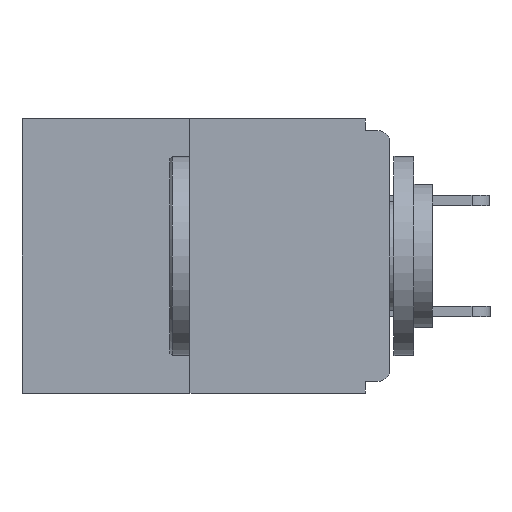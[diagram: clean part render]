
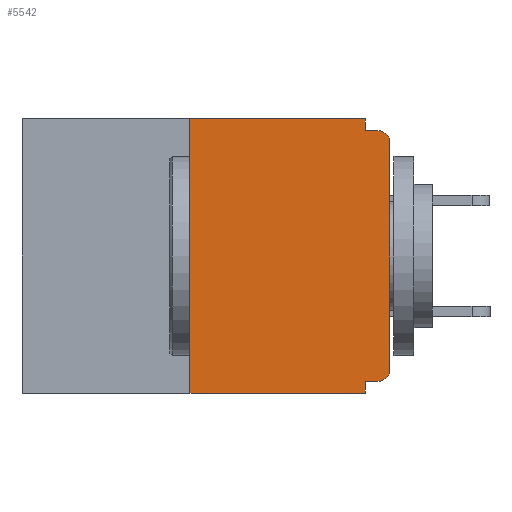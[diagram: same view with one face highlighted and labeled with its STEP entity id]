
A CAD part, left-side view. The second image highlights one B-rep face of the part: STEP entity #5542.
In plain terms, the highlighted planar face has unit normal (-1, 0, 0).
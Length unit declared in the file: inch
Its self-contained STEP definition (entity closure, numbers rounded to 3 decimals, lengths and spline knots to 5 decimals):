
#124 = DIRECTION ( 'NONE',  ( 0., 0., -1. ) ) ;
#130 = LINE ( 'NONE', #14023, #1380 ) ;
#242 = DIRECTION ( 'NONE',  ( 0., 0., 1. ) ) ;
#257 = CARTESIAN_POINT ( 'NONE',  ( 0., 0.015, -0.015 ) ) ;
#383 = CARTESIAN_POINT ( 'NONE',  ( 0., 0., -0.015 ) ) ;
#471 = ORIENTED_EDGE ( 'NONE', *, *, #10019, .T. ) ;
#706 = EDGE_CURVE ( 'NONE', #10650, #2306, #13556, .T. ) ;
#958 = CARTESIAN_POINT ( 'NONE',  ( 0., 0.015, -0.328 ) ) ;
#968 = ORIENTED_EDGE ( 'NONE', *, *, #706, .F. ) ;
#1335 = VERTEX_POINT ( 'NONE', #4681 ) ;
#1380 = VECTOR ( 'NONE', #8545, 39.37008 ) ;
#1391 = AXIS2_PLACEMENT_3D ( 'NONE', #11073, #4269, #13406 ) ;
#1446 = VERTEX_POINT ( 'NONE', #8857 ) ;
#1545 = DIRECTION ( 'NONE',  ( 0., -1., 0. ) ) ;
#1684 = DIRECTION ( 'NONE',  ( 0., 0., -1. ) ) ;
#1802 = ORIENTED_EDGE ( 'NONE', *, *, #4657, .T. ) ;
#1817 = VECTOR ( 'NONE', #9415, 39.37008 ) ;
#1826 = ORIENTED_EDGE ( 'NONE', *, *, #4753, .F. ) ;
#2058 = CARTESIAN_POINT ( 'NONE',  ( 0., 0.25, -0.343 ) ) ;
#2094 = CARTESIAN_POINT ( 'NONE',  ( 0., 0.25, 0. ) ) ;
#2144 = ORIENTED_EDGE ( 'NONE', *, *, #2941, .F. ) ;
#2306 = VERTEX_POINT ( 'NONE', #257 ) ;
#2611 = CARTESIAN_POINT ( 'NONE',  ( 0., 0.46, 0. ) ) ;
#2941 = EDGE_CURVE ( 'NONE', #1446, #10650, #130, .T. ) ;
#3149 = CARTESIAN_POINT ( 'NONE',  ( 0., 0., -0.313 ) ) ;
#3256 = ORIENTED_EDGE ( 'NONE', *, *, #12972, .T. ) ;
#3649 = DIRECTION ( 'NONE',  ( 0., 0., 1. ) ) ;
#3803 = CARTESIAN_POINT ( 'NONE',  ( 0., 0.25, 0. ) ) ;
#4005 = EDGE_CURVE ( 'NONE', #9898, #11535, #7190, .T. ) ;
#4269 = DIRECTION ( 'NONE',  ( -1., 0., 0. ) ) ;
#4468 = CIRCLE ( 'NONE', #1391, 0.015 ) ;
#4657 = EDGE_CURVE ( 'NONE', #9674, #9310, #10744, .T. ) ;
#4681 = CARTESIAN_POINT ( 'NONE',  ( 0., 0.031, -0.328 ) ) ;
#4753 = EDGE_CURVE ( 'NONE', #11618, #1335, #5361, .T. ) ;
#5146 = DIRECTION ( 'NONE',  ( 0., -1., 0. ) ) ;
#5262 = VECTOR ( 'NONE', #5146, 39.37008 ) ;
#5347 = EDGE_CURVE ( 'NONE', #9310, #2306, #4468, .T. ) ;
#5361 = LINE ( 'NONE', #10665, #1817 ) ;
#5542 = ADVANCED_FACE ( 'NONE', ( #10370 ), #13899, .F. ) ;
#5625 = VECTOR ( 'NONE', #1684, 39.37008 ) ;
#5710 = CIRCLE ( 'NONE', #9790, 0.015 ) ;
#6798 = VERTEX_POINT ( 'NONE', #12410 ) ;
#6941 = AXIS2_PLACEMENT_3D ( 'NONE', #8319, #9202, #124 ) ;
#6964 = CARTESIAN_POINT ( 'NONE',  ( 0., 0., 0. ) ) ;
#7073 = EDGE_CURVE ( 'NONE', #11535, #1446, #12800, .T. ) ;
#7163 = DIRECTION ( 'NONE',  ( 0., 0., -1. ) ) ;
#7190 = LINE ( 'NONE', #3803, #14631 ) ;
#7388 = CARTESIAN_POINT ( 'NONE',  ( 0., 0.031, -0.343 ) ) ;
#7446 = LINE ( 'NONE', #7388, #5625 ) ;
#8319 = CARTESIAN_POINT ( 'NONE',  ( 0., 0.46, 0. ) ) ;
#8545 = DIRECTION ( 'NONE',  ( 0., 0., -1. ) ) ;
#8546 = EDGE_CURVE ( 'NONE', #1335, #6798, #7446, .T. ) ;
#8857 = CARTESIAN_POINT ( 'NONE',  ( 0., 0.031, 0. ) ) ;
#9029 = ORIENTED_EDGE ( 'NONE', *, *, #7073, .F. ) ;
#9202 = DIRECTION ( 'NONE',  ( 1., 0., 0. ) ) ;
#9310 = VERTEX_POINT ( 'NONE', #10339 ) ;
#9407 = DIRECTION ( 'NONE',  ( -1., 0., 0. ) ) ;
#9415 = DIRECTION ( 'NONE',  ( 0., 1., 0. ) ) ;
#9499 = DIRECTION ( 'NONE',  ( 0., -1., 0. ) ) ;
#9599 = CARTESIAN_POINT ( 'NONE',  ( 0., 0.031, -0.015 ) ) ;
#9674 = VERTEX_POINT ( 'NONE', #3149 ) ;
#9790 = AXIS2_PLACEMENT_3D ( 'NONE', #12768, #9407, #7163 ) ;
#9816 = VECTOR ( 'NONE', #1545, 39.37008 ) ;
#9898 = VERTEX_POINT ( 'NONE', #2058 ) ;
#10019 = EDGE_CURVE ( 'NONE', #9898, #6798, #10992, .T. ) ;
#10075 = ORIENTED_EDGE ( 'NONE', *, *, #8546, .F. ) ;
#10339 = CARTESIAN_POINT ( 'NONE',  ( 0., 0., -0.03 ) ) ;
#10370 = FACE_OUTER_BOUND ( 'NONE', #10453, .T. ) ;
#10453 = EDGE_LOOP ( 'NONE', ( #9029, #13191, #471, #10075, #1826, #3256, #1802, #13804, #968, #2144 ) ) ;
#10571 = VECTOR ( 'NONE', #9499, 39.37008 ) ;
#10650 = VERTEX_POINT ( 'NONE', #9599 ) ;
#10665 = CARTESIAN_POINT ( 'NONE',  ( 0., 0., -0.328 ) ) ;
#10744 = LINE ( 'NONE', #6964, #13010 ) ;
#10992 = LINE ( 'NONE', #12798, #5262 ) ;
#11073 = CARTESIAN_POINT ( 'NONE',  ( 0., 0.015, -0.03 ) ) ;
#11535 = VERTEX_POINT ( 'NONE', #2094 ) ;
#11618 = VERTEX_POINT ( 'NONE', #958 ) ;
#12410 = CARTESIAN_POINT ( 'NONE',  ( 0., 0.031, -0.343 ) ) ;
#12768 = CARTESIAN_POINT ( 'NONE',  ( 0., 0.015, -0.313 ) ) ;
#12798 = CARTESIAN_POINT ( 'NONE',  ( 0., 0.46, -0.343 ) ) ;
#12800 = LINE ( 'NONE', #2611, #9816 ) ;
#12972 = EDGE_CURVE ( 'NONE', #11618, #9674, #5710, .T. ) ;
#13010 = VECTOR ( 'NONE', #242, 39.37008 ) ;
#13191 = ORIENTED_EDGE ( 'NONE', *, *, #4005, .F. ) ;
#13406 = DIRECTION ( 'NONE',  ( 0., 0., -1. ) ) ;
#13556 = LINE ( 'NONE', #383, #10571 ) ;
#13804 = ORIENTED_EDGE ( 'NONE', *, *, #5347, .T. ) ;
#13899 = PLANE ( 'NONE',  #6941 ) ;
#14023 = CARTESIAN_POINT ( 'NONE',  ( 0., 0.031, 0. ) ) ;
#14631 = VECTOR ( 'NONE', #3649, 39.37008 ) ;
